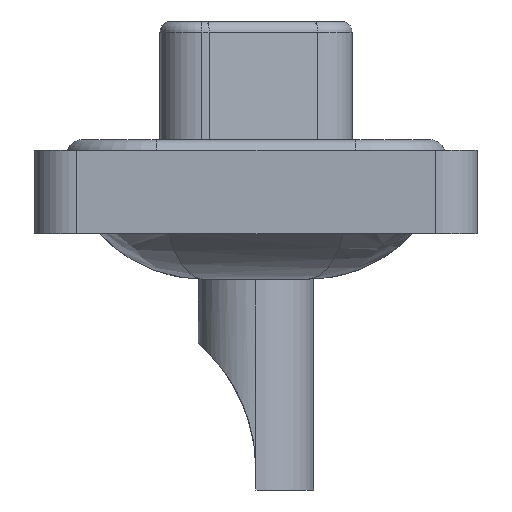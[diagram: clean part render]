
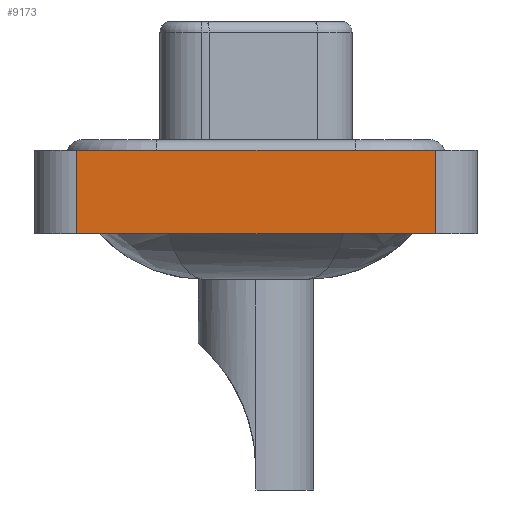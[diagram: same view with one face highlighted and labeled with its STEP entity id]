
A CAD part, left-side view. The second image highlights one B-rep face of the part: STEP entity #9173.
In plain terms, the highlighted planar face has unit normal (-1, 0, 0).
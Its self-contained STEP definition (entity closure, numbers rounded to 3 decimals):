
#149 = DIRECTION ( 'NONE',  ( 0., 0., 1. ) ) ;
#203 = VECTOR ( 'NONE', #149, 1000. ) ;
#919 = VECTOR ( 'NONE', #6544, 1000. ) ;
#1058 = CARTESIAN_POINT ( 'NONE',  ( -7.35, -8.55, -3.6 ) ) ;
#2902 = EDGE_CURVE ( 'NONE', #14006, #16081, #19922, .T. ) ;
#3027 = DIRECTION ( 'NONE',  ( 0., -1., 0. ) ) ;
#3100 = ORIENTED_EDGE ( 'NONE', *, *, #2902, .T. ) ;
#3243 = DIRECTION ( 'NONE',  ( -1., 0., 0. ) ) ;
#5278 = ORIENTED_EDGE ( 'NONE', *, *, #9962, .F. ) ;
#5634 = DIRECTION ( 'NONE',  ( 0., -1., 0. ) ) ;
#6544 = DIRECTION ( 'NONE',  ( 0., 0., 1. ) ) ;
#6613 = VERTEX_POINT ( 'NONE', #21428 ) ;
#6928 = PLANE ( 'NONE',  #19343 ) ;
#9173 = ADVANCED_FACE ( 'NONE', ( #10070 ), #6928, .T. ) ;
#9962 = EDGE_CURVE ( 'NONE', #14006, #17887, #15607, .T. ) ;
#10070 = FACE_OUTER_BOUND ( 'NONE', #11911, .T. ) ;
#10568 = CARTESIAN_POINT ( 'NONE',  ( -7.35, 8.55, -3.6 ) ) ;
#11382 = VECTOR ( 'NONE', #3027, 1000. ) ;
#11730 = CARTESIAN_POINT ( 'NONE',  ( -7.35, -8.55, -3.6 ) ) ;
#11911 = EDGE_LOOP ( 'NONE', ( #12652, #19349, #5278, #3100 ) ) ;
#11952 = CARTESIAN_POINT ( 'NONE',  ( -7.35, -8.55, -3.6 ) ) ;
#12652 = ORIENTED_EDGE ( 'NONE', *, *, #16017, .T. ) ;
#12666 = CARTESIAN_POINT ( 'NONE',  ( -7.35, -8.55, 0.4 ) ) ;
#14006 = VERTEX_POINT ( 'NONE', #21625 ) ;
#15031 = VECTOR ( 'NONE', #5634, 1000. ) ;
#15607 = LINE ( 'NONE', #10568, #203 ) ;
#16017 = EDGE_CURVE ( 'NONE', #16081, #6613, #20092, .T. ) ;
#16038 = LINE ( 'NONE', #12666, #15031 ) ;
#16081 = VERTEX_POINT ( 'NONE', #1058 ) ;
#16305 = CARTESIAN_POINT ( 'NONE',  ( -7.35, 8.55, 0.4 ) ) ;
#17887 = VERTEX_POINT ( 'NONE', #16305 ) ;
#19015 = DIRECTION ( 'NONE',  ( 0., 0., 1. ) ) ;
#19343 = AXIS2_PLACEMENT_3D ( 'NONE', #11952, #3243, #19015 ) ;
#19349 = ORIENTED_EDGE ( 'NONE', *, *, #21468, .F. ) ;
#19922 = LINE ( 'NONE', #11730, #11382 ) ;
#20092 = LINE ( 'NONE', #20202, #919 ) ;
#20202 = CARTESIAN_POINT ( 'NONE',  ( -7.35, -8.55, -3.6 ) ) ;
#21428 = CARTESIAN_POINT ( 'NONE',  ( -7.35, -8.55, 0.4 ) ) ;
#21468 = EDGE_CURVE ( 'NONE', #17887, #6613, #16038, .T. ) ;
#21625 = CARTESIAN_POINT ( 'NONE',  ( -7.35, 8.55, -3.6 ) ) ;
